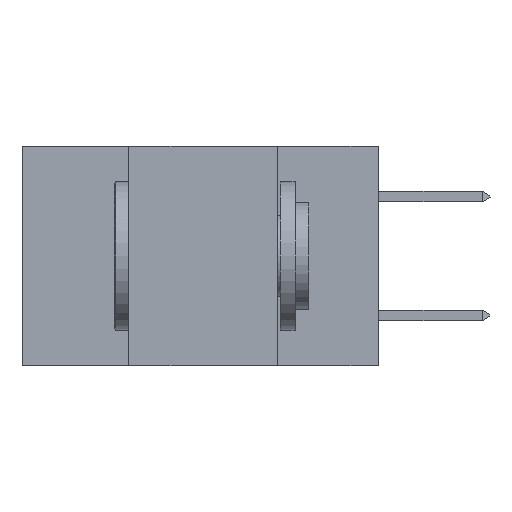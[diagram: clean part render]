
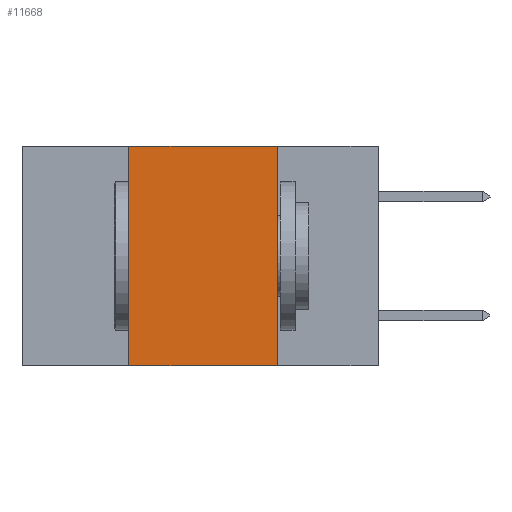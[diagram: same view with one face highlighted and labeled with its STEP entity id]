
A CAD part, left-side view. The second image highlights one B-rep face of the part: STEP entity #11668.
In plain terms, the highlighted planar face has unit normal (-1, 0, 0).
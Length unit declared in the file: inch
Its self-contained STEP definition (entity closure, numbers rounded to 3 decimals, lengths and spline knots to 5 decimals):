
#130 = CARTESIAN_POINT ( 'NONE',  ( 0., 0.42, 0. ) ) ;
#224 = VECTOR ( 'NONE', #8340, 39.37008 ) ;
#414 = DIRECTION ( 'NONE',  ( 0., 0., -1. ) ) ;
#423 = VERTEX_POINT ( 'NONE', #2559 ) ;
#611 = EDGE_CURVE ( 'NONE', #3958, #12705, #6892, .T. ) ;
#1439 = CARTESIAN_POINT ( 'NONE',  ( 0., 0.6, 0. ) ) ;
#2351 = CARTESIAN_POINT ( 'NONE',  ( 0., 0.42, -0.37 ) ) ;
#2357 = DIRECTION ( 'NONE',  ( 0., -1., 0. ) ) ;
#2559 = CARTESIAN_POINT ( 'NONE',  ( 0., 0.17, 0. ) ) ;
#2851 = ORIENTED_EDGE ( 'NONE', *, *, #6826, .F. ) ;
#2852 = FACE_OUTER_BOUND ( 'NONE', #3699, .T. ) ;
#3174 = VECTOR ( 'NONE', #12920, 39.37008 ) ;
#3521 = PLANE ( 'NONE',  #4537 ) ;
#3699 = EDGE_LOOP ( 'NONE', ( #10405, #2851, #8955, #9773 ) ) ;
#3958 = VERTEX_POINT ( 'NONE', #2351 ) ;
#4537 = AXIS2_PLACEMENT_3D ( 'NONE', #1439, #9618, #414 ) ;
#5352 = CARTESIAN_POINT ( 'NONE',  ( 0., 0.6, -0.37 ) ) ;
#6260 = CARTESIAN_POINT ( 'NONE',  ( 0., 0.17, -0.37 ) ) ;
#6826 = EDGE_CURVE ( 'NONE', #12705, #423, #9636, .T. ) ;
#6892 = LINE ( 'NONE', #10521, #8539 ) ;
#7693 = CARTESIAN_POINT ( 'NONE',  ( 0., 0.17, 0. ) ) ;
#7725 = LINE ( 'NONE', #7693, #3174 ) ;
#7963 = VERTEX_POINT ( 'NONE', #6260 ) ;
#8340 = DIRECTION ( 'NONE',  ( 0., -1., 0. ) ) ;
#8539 = VECTOR ( 'NONE', #10562, 39.37008 ) ;
#8757 = EDGE_CURVE ( 'NONE', #3958, #7963, #9595, .T. ) ;
#8955 = ORIENTED_EDGE ( 'NONE', *, *, #611, .F. ) ;
#9336 = CARTESIAN_POINT ( 'NONE',  ( 0., 0.6, 0. ) ) ;
#9595 = LINE ( 'NONE', #5352, #10725 ) ;
#9618 = DIRECTION ( 'NONE',  ( 1., 0., 0. ) ) ;
#9636 = LINE ( 'NONE', #9336, #224 ) ;
#9773 = ORIENTED_EDGE ( 'NONE', *, *, #8757, .T. ) ;
#10405 = ORIENTED_EDGE ( 'NONE', *, *, #11160, .F. ) ;
#10521 = CARTESIAN_POINT ( 'NONE',  ( 0., 0.42, 0. ) ) ;
#10562 = DIRECTION ( 'NONE',  ( 0., 0., 1. ) ) ;
#10725 = VECTOR ( 'NONE', #2357, 39.37008 ) ;
#11160 = EDGE_CURVE ( 'NONE', #423, #7963, #7725, .T. ) ;
#11668 = ADVANCED_FACE ( 'NONE', ( #2852 ), #3521, .F. ) ;
#12705 = VERTEX_POINT ( 'NONE', #130 ) ;
#12920 = DIRECTION ( 'NONE',  ( 0., 0., -1. ) ) ;
